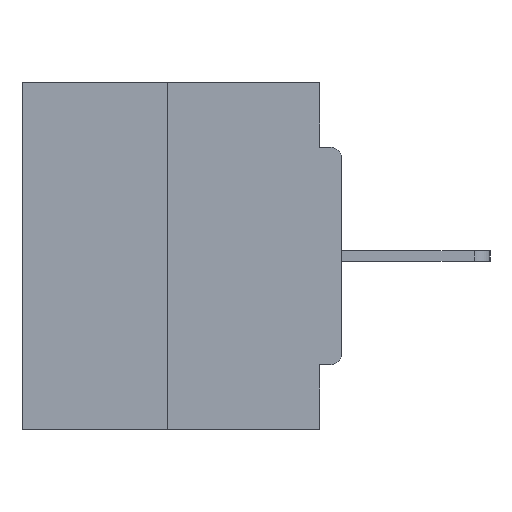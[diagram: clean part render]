
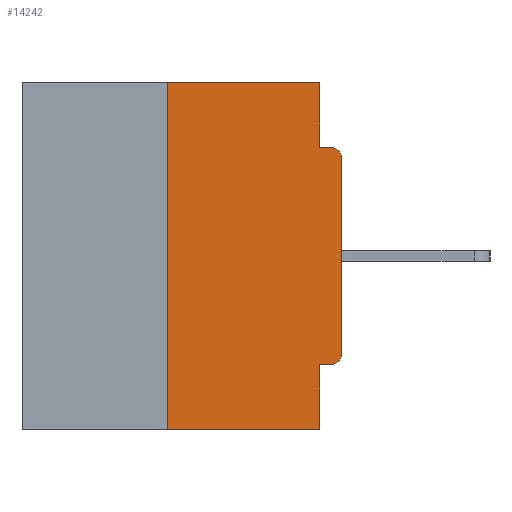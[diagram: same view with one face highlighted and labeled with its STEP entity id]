
A CAD part, left-side view. The second image highlights one B-rep face of the part: STEP entity #14242.
In plain terms, the highlighted planar face has unit normal (-1, 0, 0).
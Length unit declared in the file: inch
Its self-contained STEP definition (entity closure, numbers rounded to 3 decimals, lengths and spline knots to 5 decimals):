
#340 = EDGE_CURVE ( 'NONE', #29767, #24052, #13167, .T. ) ;
#1165 = DIRECTION ( 'NONE',  ( 0., -1., 0. ) ) ;
#1572 = AXIS2_PLACEMENT_3D ( 'NONE', #2762, #14968, #27168 ) ;
#1713 = VECTOR ( 'NONE', #11670, 39.37008 ) ;
#1939 = VERTEX_POINT ( 'NONE', #12551 ) ;
#2562 = LINE ( 'NONE', #33152, #25949 ) ;
#2737 = EDGE_CURVE ( 'NONE', #1939, #34361, #5663, .T. ) ;
#2762 = CARTESIAN_POINT ( 'NONE',  ( 0., 0.015, -0.3915 ) ) ;
#4212 = DIRECTION ( 'NONE',  ( 0., 0., -1. ) ) ;
#4718 = VERTEX_POINT ( 'NONE', #5622 ) ;
#4733 = LINE ( 'NONE', #19941, #7837 ) ;
#5622 = CARTESIAN_POINT ( 'NONE',  ( 0., 0.031, -0.5 ) ) ;
#5663 = LINE ( 'NONE', #6045, #20368 ) ;
#5755 = ORIENTED_EDGE ( 'NONE', *, *, #21307, .T. ) ;
#5766 = DIRECTION ( 'NONE',  ( 0., 0., -1. ) ) ;
#6045 = CARTESIAN_POINT ( 'NONE',  ( 0., 0., -0.4065 ) ) ;
#6208 = VECTOR ( 'NONE', #35234, 39.37008 ) ;
#6637 = CARTESIAN_POINT ( 'NONE',  ( 0., 0., -0.1085 ) ) ;
#6845 = LINE ( 'NONE', #12847, #10151 ) ;
#7837 = VECTOR ( 'NONE', #29337, 39.37008 ) ;
#8289 = VERTEX_POINT ( 'NONE', #29046 ) ;
#8449 = ORIENTED_EDGE ( 'NONE', *, *, #340, .F. ) ;
#9486 = CARTESIAN_POINT ( 'NONE',  ( 0., 0.25, -0.5 ) ) ;
#9941 = AXIS2_PLACEMENT_3D ( 'NONE', #32396, #10426, #4212 ) ;
#10151 = VECTOR ( 'NONE', #28423, 39.37008 ) ;
#10421 = ORIENTED_EDGE ( 'NONE', *, *, #2737, .F. ) ;
#10426 = DIRECTION ( 'NONE',  ( -1., 0., 0. ) ) ;
#10702 = CARTESIAN_POINT ( 'NONE',  ( 0., 0.031, 0. ) ) ;
#10717 = ORIENTED_EDGE ( 'NONE', *, *, #34096, .F. ) ;
#11670 = DIRECTION ( 'NONE',  ( 0., 0., 1. ) ) ;
#12333 = EDGE_CURVE ( 'NONE', #21259, #20812, #37592, .T. ) ;
#12551 = CARTESIAN_POINT ( 'NONE',  ( 0., 0.015, -0.4065 ) ) ;
#12770 = VECTOR ( 'NONE', #1165, 39.37008 ) ;
#12847 = CARTESIAN_POINT ( 'NONE',  ( 0., 0.46, -0.5 ) ) ;
#13167 = LINE ( 'NONE', #34147, #12770 ) ;
#13600 = CARTESIAN_POINT ( 'NONE',  ( 0., 0.015, -0.0935 ) ) ;
#13625 = EDGE_CURVE ( 'NONE', #15654, #20812, #36757, .T. ) ;
#13722 = ORIENTED_EDGE ( 'NONE', *, *, #14195, .F. ) ;
#14171 = FACE_OUTER_BOUND ( 'NONE', #35819, .T. ) ;
#14195 = EDGE_CURVE ( 'NONE', #24052, #21259, #2562, .T. ) ;
#14242 = ADVANCED_FACE ( 'NONE', ( #14171 ), #38531, .F. ) ;
#14968 = DIRECTION ( 'NONE',  ( -1., 0., 0. ) ) ;
#15654 = VERTEX_POINT ( 'NONE', #6637 ) ;
#15763 = CARTESIAN_POINT ( 'NONE',  ( 0., 0.031, -0.0935 ) ) ;
#16283 = CIRCLE ( 'NONE', #1572, 0.015 ) ;
#16803 = CARTESIAN_POINT ( 'NONE',  ( 0., 0., -0.0935 ) ) ;
#17653 = DIRECTION ( 'NONE',  ( 0., 1., 0. ) ) ;
#17681 = EDGE_CURVE ( 'NONE', #1939, #8289, #16283, .T. ) ;
#19941 = CARTESIAN_POINT ( 'NONE',  ( 0., 0., 0. ) ) ;
#20251 = VERTEX_POINT ( 'NONE', #9486 ) ;
#20368 = VECTOR ( 'NONE', #17653, 39.37008 ) ;
#20759 = CARTESIAN_POINT ( 'NONE',  ( 0., 0.46, 0. ) ) ;
#20812 = VERTEX_POINT ( 'NONE', #13600 ) ;
#20873 = ORIENTED_EDGE ( 'NONE', *, *, #17681, .T. ) ;
#21259 = VERTEX_POINT ( 'NONE', #15763 ) ;
#21307 = EDGE_CURVE ( 'NONE', #8289, #15654, #4733, .T. ) ;
#23379 = AXIS2_PLACEMENT_3D ( 'NONE', #20759, #32939, #26961 ) ;
#24052 = VERTEX_POINT ( 'NONE', #10702 ) ;
#25621 = DIRECTION ( 'NONE',  ( 0., -1., 0. ) ) ;
#25836 = LINE ( 'NONE', #29615, #6208 ) ;
#25949 = VECTOR ( 'NONE', #5766, 39.37008 ) ;
#26961 = DIRECTION ( 'NONE',  ( 0., 0., -1. ) ) ;
#27168 = DIRECTION ( 'NONE',  ( 0., 0., -1. ) ) ;
#27238 = EDGE_CURVE ( 'NONE', #34361, #4718, #25836, .T. ) ;
#27260 = LINE ( 'NONE', #39235, #1713 ) ;
#28423 = DIRECTION ( 'NONE',  ( 0., -1., 0. ) ) ;
#29046 = CARTESIAN_POINT ( 'NONE',  ( 0., 0., -0.3915 ) ) ;
#29337 = DIRECTION ( 'NONE',  ( 0., 0., 1. ) ) ;
#29615 = CARTESIAN_POINT ( 'NONE',  ( 0., 0.031, -0.5 ) ) ;
#29767 = VERTEX_POINT ( 'NONE', #38495 ) ;
#30830 = CARTESIAN_POINT ( 'NONE',  ( 0., 0.031, -0.4065 ) ) ;
#32396 = CARTESIAN_POINT ( 'NONE',  ( 0., 0.015, -0.1085 ) ) ;
#32621 = ORIENTED_EDGE ( 'NONE', *, *, #36066, .T. ) ;
#32939 = DIRECTION ( 'NONE',  ( 1., 0., 0. ) ) ;
#33152 = CARTESIAN_POINT ( 'NONE',  ( 0., 0.031, 0. ) ) ;
#33714 = ORIENTED_EDGE ( 'NONE', *, *, #12333, .F. ) ;
#34096 = EDGE_CURVE ( 'NONE', #20251, #29767, #27260, .T. ) ;
#34147 = CARTESIAN_POINT ( 'NONE',  ( 0., 0.46, 0. ) ) ;
#34361 = VERTEX_POINT ( 'NONE', #30830 ) ;
#35234 = DIRECTION ( 'NONE',  ( 0., 0., -1. ) ) ;
#35819 = EDGE_LOOP ( 'NONE', ( #8449, #10717, #32621, #37255, #10421, #20873, #5755, #38227, #33714, #13722 ) ) ;
#36066 = EDGE_CURVE ( 'NONE', #20251, #4718, #6845, .T. ) ;
#36757 = CIRCLE ( 'NONE', #9941, 0.015 ) ;
#37255 = ORIENTED_EDGE ( 'NONE', *, *, #27238, .F. ) ;
#37592 = LINE ( 'NONE', #16803, #39273 ) ;
#38227 = ORIENTED_EDGE ( 'NONE', *, *, #13625, .T. ) ;
#38495 = CARTESIAN_POINT ( 'NONE',  ( 0., 0.25, 0. ) ) ;
#38531 = PLANE ( 'NONE',  #23379 ) ;
#39235 = CARTESIAN_POINT ( 'NONE',  ( 0., 0.25, 0. ) ) ;
#39273 = VECTOR ( 'NONE', #25621, 39.37008 ) ;
